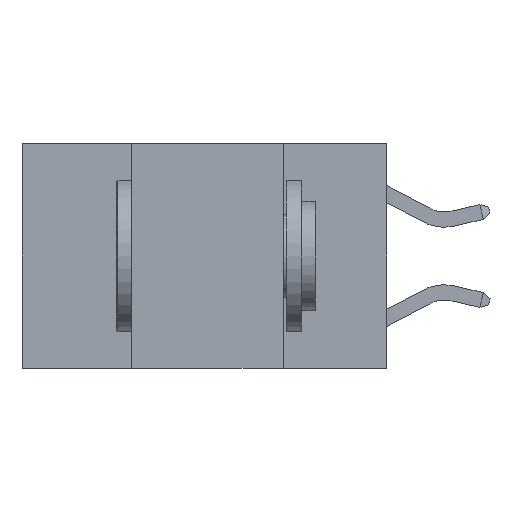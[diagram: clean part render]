
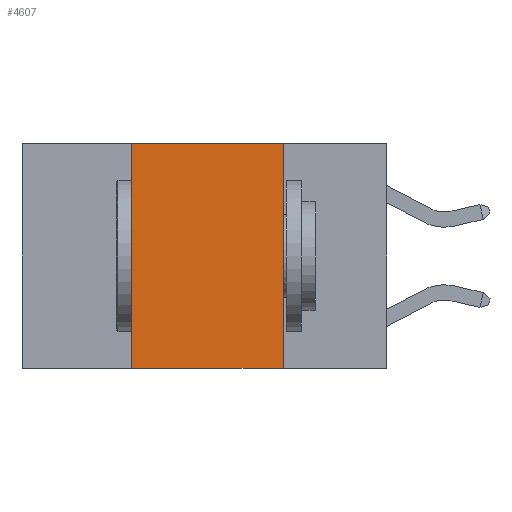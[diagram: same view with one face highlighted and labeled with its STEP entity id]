
A CAD part, left-side view. The second image highlights one B-rep face of the part: STEP entity #4607.
In plain terms, the highlighted planar face has unit normal (-1, 0, 0).
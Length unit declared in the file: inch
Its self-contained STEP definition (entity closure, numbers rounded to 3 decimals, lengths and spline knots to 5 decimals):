
#1350 = DIRECTION ( 'NONE',  ( 1., 0., 0. ) ) ;
#1742 = ORIENTED_EDGE ( 'NONE', *, *, #12002, .F. ) ;
#1854 = DIRECTION ( 'NONE',  ( 0., -1., 0. ) ) ;
#1881 = CARTESIAN_POINT ( 'NONE',  ( 0., 0.6, -0.37 ) ) ;
#2084 = DIRECTION ( 'NONE',  ( 0., 0., 1. ) ) ;
#2114 = DIRECTION ( 'NONE',  ( 0., 0., -1. ) ) ;
#2823 = VERTEX_POINT ( 'NONE', #4596 ) ;
#3004 = CARTESIAN_POINT ( 'NONE',  ( 0., 0.6, 0. ) ) ;
#3162 = EDGE_CURVE ( 'NONE', #11089, #7778, #11739, .T. ) ;
#3628 = FACE_OUTER_BOUND ( 'NONE', #7700, .T. ) ;
#3808 = EDGE_CURVE ( 'NONE', #11089, #2823, #4366, .T. ) ;
#4060 = AXIS2_PLACEMENT_3D ( 'NONE', #11569, #1350, #7946 ) ;
#4158 = ORIENTED_EDGE ( 'NONE', *, *, #3162, .T. ) ;
#4366 = LINE ( 'NONE', #7707, #9285 ) ;
#4452 = EDGE_CURVE ( 'NONE', #5811, #7778, #11869, .T. ) ;
#4596 = CARTESIAN_POINT ( 'NONE',  ( 0., 0.42, 0. ) ) ;
#4607 = ADVANCED_FACE ( 'NONE', ( #3628 ), #10693, .F. ) ;
#4679 = VECTOR ( 'NONE', #1854, 39.37008 ) ;
#5773 = VECTOR ( 'NONE', #10468, 39.37008 ) ;
#5811 = VERTEX_POINT ( 'NONE', #7988 ) ;
#6076 = LINE ( 'NONE', #3004, #5773 ) ;
#6959 = ORIENTED_EDGE ( 'NONE', *, *, #4452, .F. ) ;
#7700 = EDGE_LOOP ( 'NONE', ( #6959, #1742, #10007, #4158 ) ) ;
#7707 = CARTESIAN_POINT ( 'NONE',  ( 0., 0.42, 0. ) ) ;
#7778 = VERTEX_POINT ( 'NONE', #12033 ) ;
#7946 = DIRECTION ( 'NONE',  ( 0., 0., -1. ) ) ;
#7988 = CARTESIAN_POINT ( 'NONE',  ( 0., 0.17, 0. ) ) ;
#8030 = CARTESIAN_POINT ( 'NONE',  ( 0., 0.42, -0.37 ) ) ;
#9285 = VECTOR ( 'NONE', #2084, 39.37008 ) ;
#9580 = CARTESIAN_POINT ( 'NONE',  ( 0., 0.17, 0. ) ) ;
#10007 = ORIENTED_EDGE ( 'NONE', *, *, #3808, .F. ) ;
#10468 = DIRECTION ( 'NONE',  ( 0., -1., 0. ) ) ;
#10693 = PLANE ( 'NONE',  #4060 ) ;
#11089 = VERTEX_POINT ( 'NONE', #8030 ) ;
#11569 = CARTESIAN_POINT ( 'NONE',  ( 0., 0.6, 0. ) ) ;
#11591 = VECTOR ( 'NONE', #2114, 39.37008 ) ;
#11739 = LINE ( 'NONE', #1881, #4679 ) ;
#11869 = LINE ( 'NONE', #9580, #11591 ) ;
#12002 = EDGE_CURVE ( 'NONE', #2823, #5811, #6076, .T. ) ;
#12033 = CARTESIAN_POINT ( 'NONE',  ( 0., 0.17, -0.37 ) ) ;
